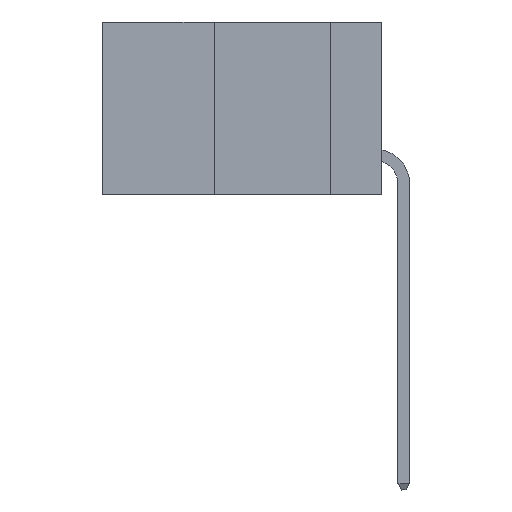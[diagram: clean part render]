
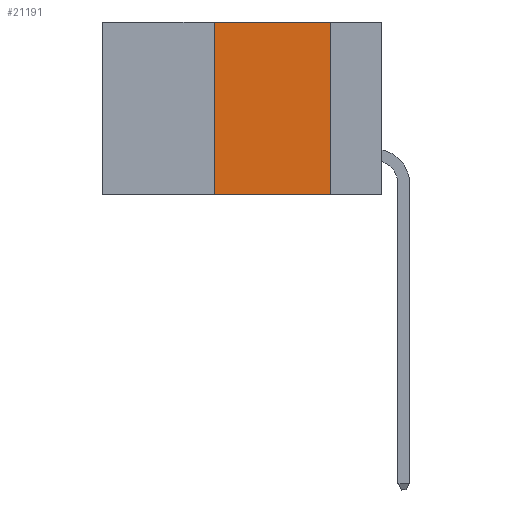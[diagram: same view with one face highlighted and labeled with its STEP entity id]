
A CAD part, left-side view. The second image highlights one B-rep face of the part: STEP entity #21191.
In plain terms, the highlighted planar face has unit normal (-1, 0, 0).
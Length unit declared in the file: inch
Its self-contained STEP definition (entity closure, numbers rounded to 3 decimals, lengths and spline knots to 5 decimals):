
#927 = DIRECTION ( 'NONE',  ( 0., 0., -1. ) ) ;
#2325 = EDGE_CURVE ( 'NONE', #12500, #21249, #16755, .T. ) ;
#3212 = DIRECTION ( 'NONE',  ( 0., -1., 0. ) ) ;
#3543 = PLANE ( 'NONE',  #33719 ) ;
#3958 = CARTESIAN_POINT ( 'NONE',  ( 0., 0.11, 0. ) ) ;
#4996 = LINE ( 'NONE', #3958, #15352 ) ;
#5069 = ORIENTED_EDGE ( 'NONE', *, *, #31084, .F. ) ;
#5749 = CARTESIAN_POINT ( 'NONE',  ( 0., 0.6, 0. ) ) ;
#6437 = DIRECTION ( 'NONE',  ( 1., 0., 0. ) ) ;
#6821 = CARTESIAN_POINT ( 'NONE',  ( 0., 0.36, -0.37 ) ) ;
#8088 = CARTESIAN_POINT ( 'NONE',  ( 0., 0.36, 0. ) ) ;
#8910 = EDGE_CURVE ( 'NONE', #21384, #21249, #4996, .T. ) ;
#9080 = EDGE_CURVE ( 'NONE', #12500, #28336, #19870, .T. ) ;
#9478 = CARTESIAN_POINT ( 'NONE',  ( 0., 0.11, 0. ) ) ;
#10001 = VECTOR ( 'NONE', #33373, 39.37008 ) ;
#10548 = VECTOR ( 'NONE', #3212, 39.37008 ) ;
#11535 = DIRECTION ( 'NONE',  ( 0., 0., -1. ) ) ;
#12500 = VERTEX_POINT ( 'NONE', #6821 ) ;
#13620 = DIRECTION ( 'NONE',  ( 0., -1., 0. ) ) ;
#13753 = ORIENTED_EDGE ( 'NONE', *, *, #9080, .F. ) ;
#13881 = CARTESIAN_POINT ( 'NONE',  ( 0., 0.6, -0.37 ) ) ;
#15352 = VECTOR ( 'NONE', #927, 39.37008 ) ;
#16755 = LINE ( 'NONE', #13881, #10548 ) ;
#17464 = ORIENTED_EDGE ( 'NONE', *, *, #8910, .F. ) ;
#19717 = CARTESIAN_POINT ( 'NONE',  ( 0., 0.11, -0.37 ) ) ;
#19870 = LINE ( 'NONE', #22753, #10001 ) ;
#21191 = ADVANCED_FACE ( 'NONE', ( #26789 ), #3543, .F. ) ;
#21249 = VERTEX_POINT ( 'NONE', #19717 ) ;
#21384 = VERTEX_POINT ( 'NONE', #9478 ) ;
#22753 = CARTESIAN_POINT ( 'NONE',  ( 0., 0.36, 0. ) ) ;
#24793 = ORIENTED_EDGE ( 'NONE', *, *, #2325, .T. ) ;
#24873 = VECTOR ( 'NONE', #13620, 39.37008 ) ;
#26789 = FACE_OUTER_BOUND ( 'NONE', #28143, .T. ) ;
#28143 = EDGE_LOOP ( 'NONE', ( #17464, #5069, #13753, #24793 ) ) ;
#28336 = VERTEX_POINT ( 'NONE', #8088 ) ;
#30025 = CARTESIAN_POINT ( 'NONE',  ( 0., 0.6, 0. ) ) ;
#30222 = LINE ( 'NONE', #5749, #24873 ) ;
#31084 = EDGE_CURVE ( 'NONE', #28336, #21384, #30222, .T. ) ;
#33373 = DIRECTION ( 'NONE',  ( 0., 0., 1. ) ) ;
#33719 = AXIS2_PLACEMENT_3D ( 'NONE', #30025, #6437, #11535 ) ;
